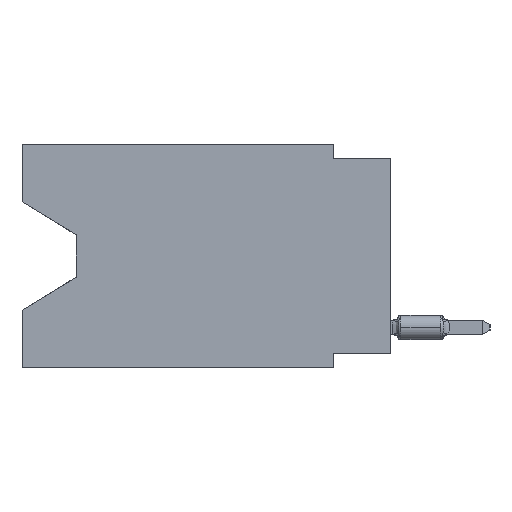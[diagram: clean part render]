
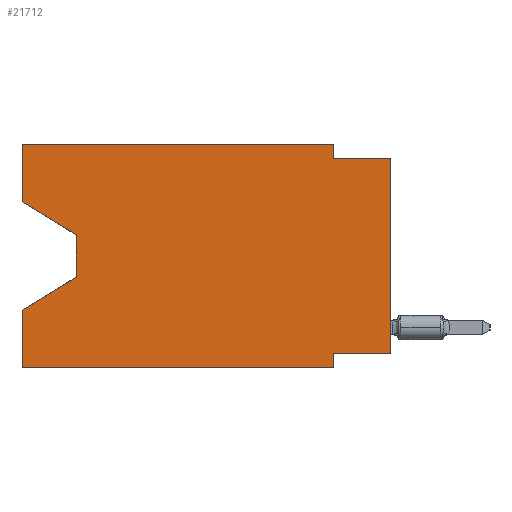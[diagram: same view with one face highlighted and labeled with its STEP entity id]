
A CAD part, left-side view. The second image highlights one B-rep face of the part: STEP entity #21712.
In plain terms, the highlighted planar face has unit normal (-1, 0, 0).
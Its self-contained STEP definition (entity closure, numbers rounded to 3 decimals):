
#109 = ORIENTED_EDGE ( 'NONE', *, *, #33374, .F. ) ;
#313 = EDGE_LOOP ( 'NONE', ( #14489, #27973, #595, #1837, #9482, #109, #13120, #349, #12021, #31515, #36160, #18809 ) ) ;
#349 = ORIENTED_EDGE ( 'NONE', *, *, #27397, .T. ) ;
#550 = VECTOR ( 'NONE', #32913, 1000. ) ;
#595 = ORIENTED_EDGE ( 'NONE', *, *, #2189, .T. ) ;
#877 = CARTESIAN_POINT ( 'NONE',  ( 0., 16.383, 0. ) ) ;
#1037 = CARTESIAN_POINT ( 'NONE',  ( 0., 2.54, 0. ) ) ;
#1837 = ORIENTED_EDGE ( 'NONE', *, *, #15926, .F. ) ;
#2002 = CARTESIAN_POINT ( 'NONE',  ( 0., 2.54, -9.906 ) ) ;
#2189 = EDGE_CURVE ( 'NONE', #15359, #8438, #33264, .T. ) ;
#2207 = VERTEX_POINT ( 'NONE', #12249 ) ;
#2295 = VECTOR ( 'NONE', #14596, 1000. ) ;
#2839 = LINE ( 'NONE', #35826, #11691 ) ;
#3075 = DIRECTION ( 'NONE',  ( 1., 0., 0. ) ) ;
#3652 = CARTESIAN_POINT ( 'NONE',  ( 0., 0., -9.271 ) ) ;
#3659 = PLANE ( 'NONE',  #7358 ) ;
#3718 = DIRECTION ( 'NONE',  ( 0., -1., 0. ) ) ;
#4503 = EDGE_CURVE ( 'NONE', #31647, #24106, #17895, .T. ) ;
#5373 = CARTESIAN_POINT ( 'NONE',  ( 0., 13.97, -4.013 ) ) ;
#5569 = CARTESIAN_POINT ( 'NONE',  ( 0., 16.383, 0. ) ) ;
#6598 = CARTESIAN_POINT ( 'NONE',  ( 0., 2.54, 0. ) ) ;
#7358 = AXIS2_PLACEMENT_3D ( 'NONE', #15243, #3075, #27229 ) ;
#7706 = LINE ( 'NONE', #2002, #20760 ) ;
#8438 = VERTEX_POINT ( 'NONE', #37484 ) ;
#8474 = CARTESIAN_POINT ( 'NONE',  ( 0., 16.383, -2.546 ) ) ;
#9482 = ORIENTED_EDGE ( 'NONE', *, *, #38804, .T. ) ;
#10124 = CARTESIAN_POINT ( 'NONE',  ( 0., 16.383, -2.546 ) ) ;
#10638 = EDGE_CURVE ( 'NONE', #31647, #25939, #2839, .T. ) ;
#11266 = EDGE_CURVE ( 'NONE', #28185, #30306, #21291, .T. ) ;
#11312 = VECTOR ( 'NONE', #14410, 1000. ) ;
#11691 = VECTOR ( 'NONE', #26603, 1000. ) ;
#11993 = CARTESIAN_POINT ( 'NONE',  ( 0., 0., -0.635 ) ) ;
#12021 = ORIENTED_EDGE ( 'NONE', *, *, #11266, .F. ) ;
#12045 = EDGE_CURVE ( 'NONE', #23421, #31368, #30359, .T. ) ;
#12059 = DIRECTION ( 'NONE',  ( 0., -1., 0. ) ) ;
#12249 = CARTESIAN_POINT ( 'NONE',  ( 0., 16.383, -9.906 ) ) ;
#12602 = VECTOR ( 'NONE', #3718, 1000. ) ;
#13120 = ORIENTED_EDGE ( 'NONE', *, *, #12045, .F. ) ;
#13975 = DIRECTION ( 'NONE',  ( 0., 0., -1. ) ) ;
#14075 = EDGE_CURVE ( 'NONE', #24807, #28185, #27028, .T. ) ;
#14410 = DIRECTION ( 'NONE',  ( 0., 0., -1. ) ) ;
#14489 = ORIENTED_EDGE ( 'NONE', *, *, #4503, .T. ) ;
#14596 = DIRECTION ( 'NONE',  ( 0., -1., 0. ) ) ;
#15237 = VECTOR ( 'NONE', #18355, 1000. ) ;
#15243 = CARTESIAN_POINT ( 'NONE',  ( 0., 16.383, 0. ) ) ;
#15359 = VERTEX_POINT ( 'NONE', #33457 ) ;
#15926 = EDGE_CURVE ( 'NONE', #2207, #8438, #33861, .T. ) ;
#17415 = VECTOR ( 'NONE', #12059, 1000. ) ;
#17895 = LINE ( 'NONE', #8474, #29087 ) ;
#18351 = CARTESIAN_POINT ( 'NONE',  ( 0., 0., -0.635 ) ) ;
#18355 = DIRECTION ( 'NONE',  ( 0., 0.855, -0.519 ) ) ;
#18809 = ORIENTED_EDGE ( 'NONE', *, *, #10638, .F. ) ;
#20760 = VECTOR ( 'NONE', #13975, 1000. ) ;
#21291 = LINE ( 'NONE', #18351, #17415 ) ;
#21712 = ADVANCED_FACE ( 'NONE', ( #30556 ), #3659, .F. ) ;
#21772 = VECTOR ( 'NONE', #38350, 1000. ) ;
#22719 = CARTESIAN_POINT ( 'NONE',  ( 0., 2.54, -9.906 ) ) ;
#23091 = CARTESIAN_POINT ( 'NONE',  ( 0., 2.54, -9.271 ) ) ;
#23421 = VERTEX_POINT ( 'NONE', #24404 ) ;
#23427 = LINE ( 'NONE', #5569, #2295 ) ;
#24106 = VERTEX_POINT ( 'NONE', #37827 ) ;
#24404 = CARTESIAN_POINT ( 'NONE',  ( 0., 0., -9.271 ) ) ;
#24573 = EDGE_CURVE ( 'NONE', #25939, #24807, #23427, .T. ) ;
#24807 = VERTEX_POINT ( 'NONE', #1037 ) ;
#25257 = VECTOR ( 'NONE', #27376, 1000. ) ;
#25696 = VERTEX_POINT ( 'NONE', #22719 ) ;
#25939 = VERTEX_POINT ( 'NONE', #34609 ) ;
#26603 = DIRECTION ( 'NONE',  ( 0., 0., 1. ) ) ;
#26727 = DIRECTION ( 'NONE',  ( 0., -0.855, -0.519 ) ) ;
#27028 = LINE ( 'NONE', #6598, #550 ) ;
#27229 = DIRECTION ( 'NONE',  ( 0., 0., -1. ) ) ;
#27376 = DIRECTION ( 'NONE',  ( 0., 0., 1. ) ) ;
#27397 = EDGE_CURVE ( 'NONE', #23421, #30306, #32454, .T. ) ;
#27973 = ORIENTED_EDGE ( 'NONE', *, *, #33051, .T. ) ;
#28185 = VERTEX_POINT ( 'NONE', #29362 ) ;
#29087 = VECTOR ( 'NONE', #26727, 1000. ) ;
#29362 = CARTESIAN_POINT ( 'NONE',  ( 0., 2.54, -0.635 ) ) ;
#30306 = VERTEX_POINT ( 'NONE', #11993 ) ;
#30359 = LINE ( 'NONE', #3652, #31271 ) ;
#30556 = FACE_OUTER_BOUND ( 'NONE', #313, .T. ) ;
#30616 = LINE ( 'NONE', #31012, #12602 ) ;
#31012 = CARTESIAN_POINT ( 'NONE',  ( 0., 16.383, -9.906 ) ) ;
#31271 = VECTOR ( 'NONE', #32911, 1000. ) ;
#31368 = VERTEX_POINT ( 'NONE', #23091 ) ;
#31515 = ORIENTED_EDGE ( 'NONE', *, *, #14075, .F. ) ;
#31647 = VERTEX_POINT ( 'NONE', #10124 ) ;
#32280 = LINE ( 'NONE', #5373, #11312 ) ;
#32454 = LINE ( 'NONE', #38540, #21772 ) ;
#32911 = DIRECTION ( 'NONE',  ( 0., 1., 0. ) ) ;
#32913 = DIRECTION ( 'NONE',  ( 0., 0., -1. ) ) ;
#33051 = EDGE_CURVE ( 'NONE', #24106, #15359, #32280, .T. ) ;
#33264 = LINE ( 'NONE', #36613, #15237 ) ;
#33374 = EDGE_CURVE ( 'NONE', #31368, #25696, #7706, .T. ) ;
#33457 = CARTESIAN_POINT ( 'NONE',  ( 0., 13.97, -5.893 ) ) ;
#33861 = LINE ( 'NONE', #877, #25257 ) ;
#34609 = CARTESIAN_POINT ( 'NONE',  ( 0., 16.383, 0. ) ) ;
#35826 = CARTESIAN_POINT ( 'NONE',  ( 0., 16.383, 0. ) ) ;
#36160 = ORIENTED_EDGE ( 'NONE', *, *, #24573, .F. ) ;
#36613 = CARTESIAN_POINT ( 'NONE',  ( 0., 13.97, -5.893 ) ) ;
#37484 = CARTESIAN_POINT ( 'NONE',  ( 0., 16.383, -7.36 ) ) ;
#37827 = CARTESIAN_POINT ( 'NONE',  ( 0., 13.97, -4.013 ) ) ;
#38350 = DIRECTION ( 'NONE',  ( 0., 0., 1. ) ) ;
#38540 = CARTESIAN_POINT ( 'NONE',  ( 0., 0., 0. ) ) ;
#38804 = EDGE_CURVE ( 'NONE', #2207, #25696, #30616, .T. ) ;
